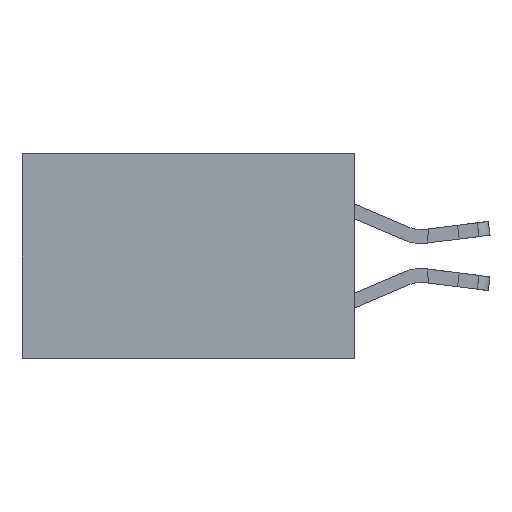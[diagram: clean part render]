
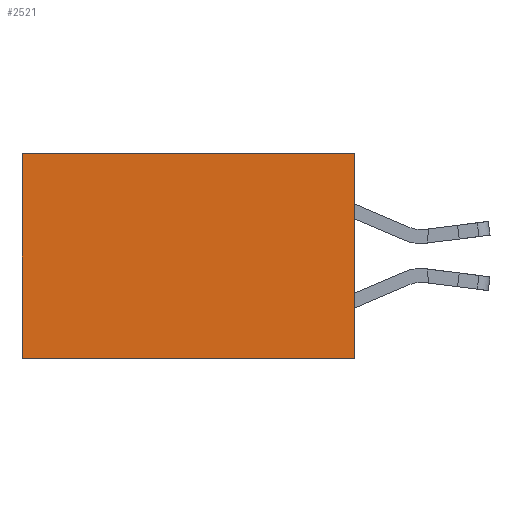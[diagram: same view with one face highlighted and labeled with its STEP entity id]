
A CAD part, left-side view. The second image highlights one B-rep face of the part: STEP entity #2521.
In plain terms, the highlighted planar face has unit normal (-1, 0, 0).
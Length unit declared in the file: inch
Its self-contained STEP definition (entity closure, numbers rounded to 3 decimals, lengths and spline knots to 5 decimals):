
#106 = CARTESIAN_POINT ( 'NONE',  ( 0.2615, 0.6, -0.37 ) ) ;
#212 = DIRECTION ( 'NONE',  ( 0., 1., 0. ) ) ;
#374 = AXIS2_PLACEMENT_3D ( 'NONE', #12655, #5601, #9301 ) ;
#1302 = LINE ( 'NONE', #4877, #4536 ) ;
#2401 = EDGE_CURVE ( 'NONE', #15191, #20280, #11087, .T. ) ;
#2521 = ADVANCED_FACE ( 'NONE', ( #14655 ), #9526, .F. ) ;
#2632 = VECTOR ( 'NONE', #22210, 39.37008 ) ;
#2644 = EDGE_LOOP ( 'NONE', ( #10212, #10446, #7727, #20957 ) ) ;
#4536 = VECTOR ( 'NONE', #23041, 39.37008 ) ;
#4587 = VECTOR ( 'NONE', #212, 39.37008 ) ;
#4877 = CARTESIAN_POINT ( 'NONE',  ( 0.2615, 0., -0.37 ) ) ;
#5123 = VERTEX_POINT ( 'NONE', #17623 ) ;
#5494 = LINE ( 'NONE', #106, #2632 ) ;
#5601 = DIRECTION ( 'NONE',  ( 1., 0., 0. ) ) ;
#7210 = CARTESIAN_POINT ( 'NONE',  ( 0.2615, 0., -0.37 ) ) ;
#7727 = ORIENTED_EDGE ( 'NONE', *, *, #15694, .F. ) ;
#8931 = VERTEX_POINT ( 'NONE', #13538 ) ;
#9301 = DIRECTION ( 'NONE',  ( 0., 0., -1. ) ) ;
#9526 = PLANE ( 'NONE',  #374 ) ;
#10212 = ORIENTED_EDGE ( 'NONE', *, *, #14039, .T. ) ;
#10446 = ORIENTED_EDGE ( 'NONE', *, *, #17666, .F. ) ;
#11087 = LINE ( 'NONE', #12996, #4587 ) ;
#11373 = LINE ( 'NONE', #7210, #12625 ) ;
#12625 = VECTOR ( 'NONE', #21691, 39.37008 ) ;
#12655 = CARTESIAN_POINT ( 'NONE',  ( 0.2615, 0., -0.37 ) ) ;
#12856 = CARTESIAN_POINT ( 'NONE',  ( 0.2615, 0.6, 0. ) ) ;
#12996 = CARTESIAN_POINT ( 'NONE',  ( 0.2615, 0., 0. ) ) ;
#13538 = CARTESIAN_POINT ( 'NONE',  ( 0.2615, 0., -0.37 ) ) ;
#14039 = EDGE_CURVE ( 'NONE', #20280, #5123, #5494, .T. ) ;
#14418 = CARTESIAN_POINT ( 'NONE',  ( 0.2615, 0., 0. ) ) ;
#14655 = FACE_OUTER_BOUND ( 'NONE', #2644, .T. ) ;
#15191 = VERTEX_POINT ( 'NONE', #14418 ) ;
#15694 = EDGE_CURVE ( 'NONE', #15191, #8931, #1302, .T. ) ;
#17623 = CARTESIAN_POINT ( 'NONE',  ( 0.2615, 0.6, -0.37 ) ) ;
#17666 = EDGE_CURVE ( 'NONE', #8931, #5123, #11373, .T. ) ;
#20280 = VERTEX_POINT ( 'NONE', #12856 ) ;
#20957 = ORIENTED_EDGE ( 'NONE', *, *, #2401, .T. ) ;
#21691 = DIRECTION ( 'NONE',  ( 0., 1., 0. ) ) ;
#22210 = DIRECTION ( 'NONE',  ( 0., 0., -1. ) ) ;
#23041 = DIRECTION ( 'NONE',  ( 0., 0., -1. ) ) ;
